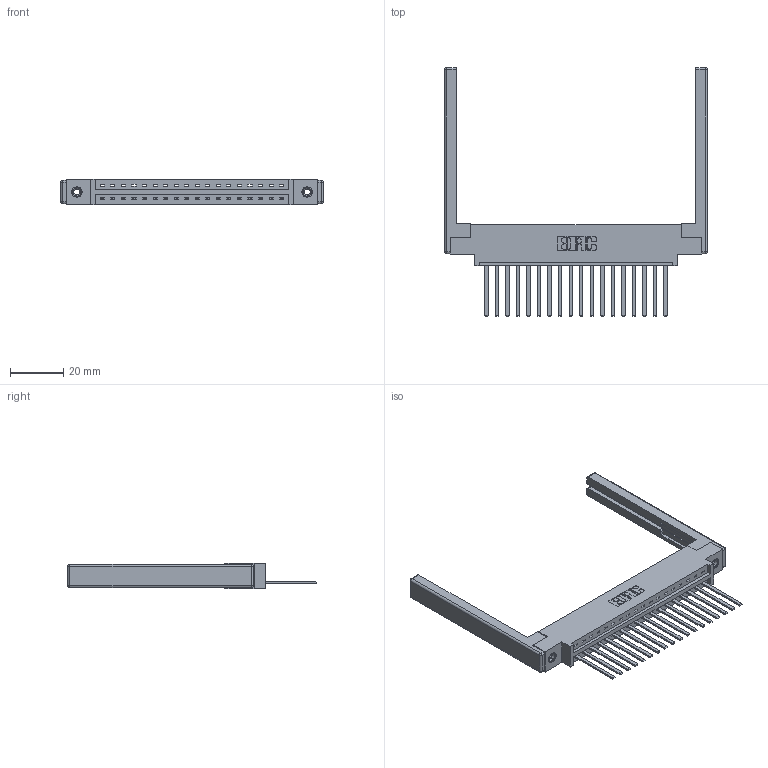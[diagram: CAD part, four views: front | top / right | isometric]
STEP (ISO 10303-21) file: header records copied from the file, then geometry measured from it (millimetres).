
FILE_DESCRIPTION (( 'STEP AP203' ), '1' );
FILE_NAME ('387-018-544-668.STEP', '2019-10-02T20:42:19', ( '' ), ( '' ), 'SwSTEP 2.0', 'SolidWorks 2016', '' );
FILE_SCHEMA (( 'CONFIG_CONTROL_DESIGN' ));
Length unit declared in the file: inch
Products named in the file (5): 345-292-001_345-293-144; 387-018-544-668; 307-220-068; 337 Part_0.170 Offset - 0.156 Dia-TI; 345-250-001_345-250-001-102
Assembly tree (23 placements, depth 2):
  387-018-544-668
    337 Part_0.170 Offset - 0.156 Dia-TI
    345-292-001_345-293-144  x18
    345-250-001_345-250-001-102  x2
    307-220-068  x2
Bounding box: 98.76 x 93.35 x 9.4 mm (x, y, z)
Volume: 14445.8 mm3; surface area: 15131.6 mm2
Topology: 23 solids, 23 shells, 1280 faces, 3773 edges, 2470 vertices
Faces by surface type: plane 918, cylinder 338, cone 12, sphere 8, torus 4
Entity records: 19192 total; most frequent: CARTESIAN_POINT 3297, ORIENTED_EDGE 3240, DIRECTION 2894, EDGE_CURVE 1620, LINE 1446, VECTOR 1446, VERTEX_POINT 1070, AXIS2_PLACEMENT_3D 724
